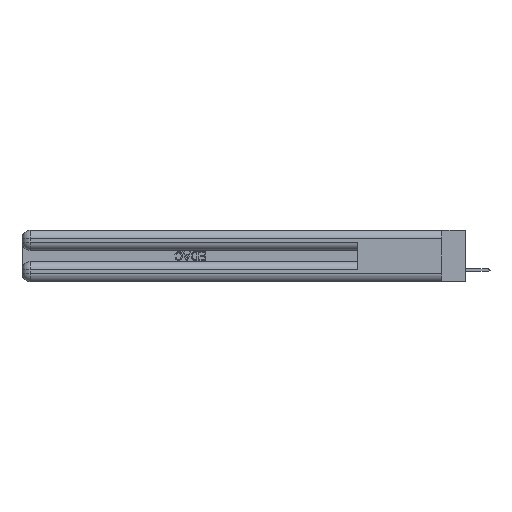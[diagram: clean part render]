
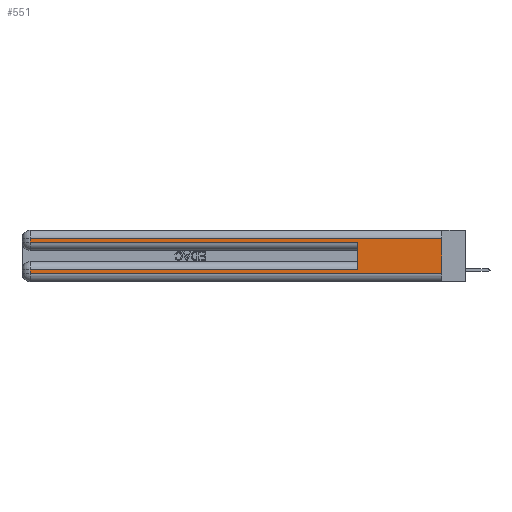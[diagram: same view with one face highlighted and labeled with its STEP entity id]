
A CAD part, left-side view. The second image highlights one B-rep face of the part: STEP entity #551.
In plain terms, the highlighted planar face has unit normal (-1, 0, 0).
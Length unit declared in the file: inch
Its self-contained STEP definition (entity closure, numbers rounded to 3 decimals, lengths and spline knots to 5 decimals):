
#231 = CARTESIAN_POINT ( 'NONE',  ( 0., 0.6, 0.085 ) ) ;
#391 = CARTESIAN_POINT ( 'NONE',  ( 0., 2.94, 0.06 ) ) ;
#551 = ADVANCED_FACE ( 'NONE', ( #35482 ), #30725, .F. ) ;
#1482 = ORIENTED_EDGE ( 'NONE', *, *, #21475, .T. ) ;
#1588 = LINE ( 'NONE', #11190, #24670 ) ;
#1749 = DIRECTION ( 'NONE',  ( 0., -1., 0. ) ) ;
#2641 = DIRECTION ( 'NONE',  ( 0., 0., -1. ) ) ;
#2774 = LINE ( 'NONE', #10902, #25387 ) ;
#3226 = EDGE_CURVE ( 'NONE', #37391, #28237, #27932, .T. ) ;
#3504 = CARTESIAN_POINT ( 'NONE',  ( 0., 0.6, 0.285 ) ) ;
#3740 = CARTESIAN_POINT ( 'NONE',  ( 0., 2.94, 0.285 ) ) ;
#4855 = EDGE_CURVE ( 'NONE', #31888, #15338, #23586, .T. ) ;
#7369 = VECTOR ( 'NONE', #13312, 39.37008 ) ;
#9274 = CARTESIAN_POINT ( 'NONE',  ( 0., 0., 0.285 ) ) ;
#9678 = ORIENTED_EDGE ( 'NONE', *, *, #33146, .F. ) ;
#10352 = CARTESIAN_POINT ( 'NONE',  ( 0., 0., 0.31 ) ) ;
#10691 = LINE ( 'NONE', #34781, #37522 ) ;
#10902 = CARTESIAN_POINT ( 'NONE',  ( 0., 0., 0.085 ) ) ;
#11190 = CARTESIAN_POINT ( 'NONE',  ( 0., 2.94, 0.37 ) ) ;
#11911 = DIRECTION ( 'NONE',  ( 0., 1., 0. ) ) ;
#12001 = DIRECTION ( 'NONE',  ( 0., -1., 0. ) ) ;
#12513 = LINE ( 'NONE', #23420, #20850 ) ;
#12585 = CARTESIAN_POINT ( 'NONE',  ( 0., 0., 0.06 ) ) ;
#12715 = DIRECTION ( 'NONE',  ( 1., 0., 0. ) ) ;
#13312 = DIRECTION ( 'NONE',  ( 0., 0., 1. ) ) ;
#13822 = DIRECTION ( 'NONE',  ( 0., 1., 0. ) ) ;
#14021 = EDGE_CURVE ( 'NONE', #18692, #16640, #1588, .T. ) ;
#15338 = VERTEX_POINT ( 'NONE', #3504 ) ;
#15858 = CARTESIAN_POINT ( 'NONE',  ( 0., 0., 0.37 ) ) ;
#15912 = ORIENTED_EDGE ( 'NONE', *, *, #3226, .T. ) ;
#16640 = VERTEX_POINT ( 'NONE', #391 ) ;
#17087 = CARTESIAN_POINT ( 'NONE',  ( 0., 0., 0.31 ) ) ;
#17167 = DIRECTION ( 'NONE',  ( 0., 0., -1. ) ) ;
#18165 = CARTESIAN_POINT ( 'NONE',  ( 0., 2.94, 0.085 ) ) ;
#18692 = VERTEX_POINT ( 'NONE', #18165 ) ;
#19445 = CARTESIAN_POINT ( 'NONE',  ( 0., 0., 0.06 ) ) ;
#19986 = ORIENTED_EDGE ( 'NONE', *, *, #25201, .T. ) ;
#20446 = VERTEX_POINT ( 'NONE', #3740 ) ;
#20850 = VECTOR ( 'NONE', #2641, 39.37008 ) ;
#20983 = EDGE_LOOP ( 'NONE', ( #9678, #15912, #19986, #33469, #36183, #1482, #33800, #27840 ) ) ;
#21475 = EDGE_CURVE ( 'NONE', #31888, #18692, #2774, .T. ) ;
#21784 = EDGE_CURVE ( 'NONE', #16640, #30993, #23953, .T. ) ;
#23112 = CARTESIAN_POINT ( 'NONE',  ( 0., 2.94, 0.31 ) ) ;
#23420 = CARTESIAN_POINT ( 'NONE',  ( 0., 0., 0.37 ) ) ;
#23586 = LINE ( 'NONE', #30653, #7369 ) ;
#23953 = LINE ( 'NONE', #19445, #36946 ) ;
#24670 = VECTOR ( 'NONE', #17167, 39.37008 ) ;
#24716 = EDGE_CURVE ( 'NONE', #20446, #15338, #37513, .T. ) ;
#25201 = EDGE_CURVE ( 'NONE', #28237, #20446, #10691, .T. ) ;
#25387 = VECTOR ( 'NONE', #11911, 39.37008 ) ;
#27840 = ORIENTED_EDGE ( 'NONE', *, *, #21784, .T. ) ;
#27932 = LINE ( 'NONE', #17087, #34872 ) ;
#28237 = VERTEX_POINT ( 'NONE', #23112 ) ;
#30653 = CARTESIAN_POINT ( 'NONE',  ( 0., 0.6, 0.145 ) ) ;
#30725 = PLANE ( 'NONE',  #33002 ) ;
#30993 = VERTEX_POINT ( 'NONE', #12585 ) ;
#31888 = VERTEX_POINT ( 'NONE', #231 ) ;
#32900 = VECTOR ( 'NONE', #12001, 39.37008 ) ;
#33002 = AXIS2_PLACEMENT_3D ( 'NONE', #15858, #12715, #33454 ) ;
#33146 = EDGE_CURVE ( 'NONE', #37391, #30993, #12513, .T. ) ;
#33454 = DIRECTION ( 'NONE',  ( 0., 0., -1. ) ) ;
#33469 = ORIENTED_EDGE ( 'NONE', *, *, #24716, .T. ) ;
#33800 = ORIENTED_EDGE ( 'NONE', *, *, #14021, .T. ) ;
#34293 = DIRECTION ( 'NONE',  ( 0., 0., -1. ) ) ;
#34781 = CARTESIAN_POINT ( 'NONE',  ( 0., 2.94, 0.37 ) ) ;
#34872 = VECTOR ( 'NONE', #13822, 39.37008 ) ;
#35482 = FACE_OUTER_BOUND ( 'NONE', #20983, .T. ) ;
#36183 = ORIENTED_EDGE ( 'NONE', *, *, #4855, .F. ) ;
#36946 = VECTOR ( 'NONE', #1749, 39.37008 ) ;
#37391 = VERTEX_POINT ( 'NONE', #10352 ) ;
#37513 = LINE ( 'NONE', #9274, #32900 ) ;
#37522 = VECTOR ( 'NONE', #34293, 39.37008 ) ;
